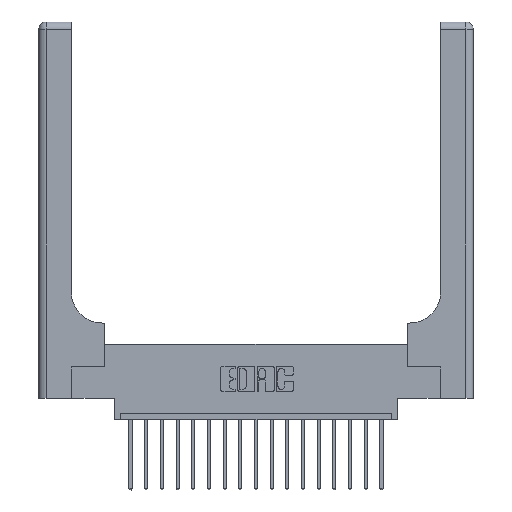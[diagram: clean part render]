
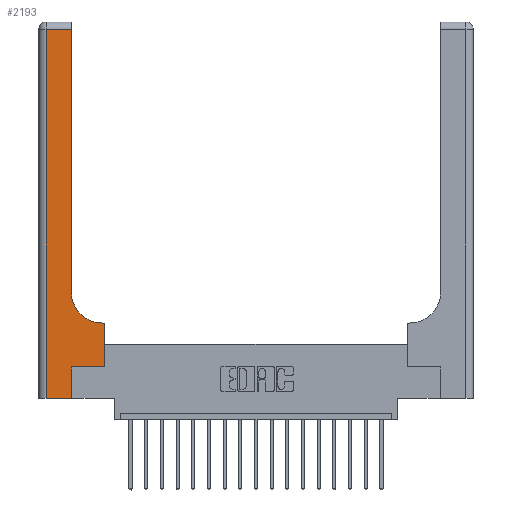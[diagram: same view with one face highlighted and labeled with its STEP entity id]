
A CAD part, top view. The second image highlights one B-rep face of the part: STEP entity #2193.
In plain terms, the highlighted planar face has unit normal (0, 0, 1).
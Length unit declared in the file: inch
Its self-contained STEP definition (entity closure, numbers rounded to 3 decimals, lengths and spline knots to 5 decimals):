
#45 = EDGE_CURVE ( 'NONE', #14187, #7645, #11312, .T. ) ;
#252 = CARTESIAN_POINT ( 'NONE',  ( 0.06, 3., 0.37 ) ) ;
#544 = EDGE_CURVE ( 'NONE', #1887, #4489, #12196, .T. ) ;
#926 = LINE ( 'NONE', #252, #4419 ) ;
#1723 = LINE ( 'NONE', #17283, #16121 ) ;
#1765 = EDGE_CURVE ( 'NONE', #5808, #10718, #11257, .T. ) ;
#1887 = VERTEX_POINT ( 'NONE', #8858 ) ;
#2193 = ADVANCED_FACE ( 'NONE', ( #14904 ), #18924, .F. ) ;
#2476 = CARTESIAN_POINT ( 'NONE',  ( 0.06, 2.94, 0.37 ) ) ;
#2919 = ORIENTED_EDGE ( 'NONE', *, *, #11813, .T. ) ;
#2943 = EDGE_CURVE ( 'NONE', #10911, #1887, #12102, .T. ) ;
#3172 = EDGE_CURVE ( 'NONE', #7645, #10911, #13008, .T. ) ;
#3522 = DIRECTION ( 'NONE',  ( 0., 1., 0. ) ) ;
#3630 = ORIENTED_EDGE ( 'NONE', *, *, #16964, .T. ) ;
#3651 = VECTOR ( 'NONE', #7905, 39.37008 ) ;
#3683 = CARTESIAN_POINT ( 'NONE',  ( 0.528, 0.25, 0.37 ) ) ;
#4224 = ORIENTED_EDGE ( 'NONE', *, *, #544, .T. ) ;
#4419 = VECTOR ( 'NONE', #13472, 39.37008 ) ;
#4489 = VERTEX_POINT ( 'NONE', #5322 ) ;
#4621 = VECTOR ( 'NONE', #13363, 39.37008 ) ;
#4865 = VECTOR ( 'NONE', #3522, 39.37008 ) ;
#4962 = CARTESIAN_POINT ( 'NONE',  ( 0.528, 0.25, 0.37 ) ) ;
#5295 = VERTEX_POINT ( 'NONE', #5803 ) ;
#5322 = CARTESIAN_POINT ( 'NONE',  ( 0.51, 0.6, 0.37 ) ) ;
#5636 = ORIENTED_EDGE ( 'NONE', *, *, #9263, .T. ) ;
#5675 = VECTOR ( 'NONE', #7975, 39.37008 ) ;
#5803 = CARTESIAN_POINT ( 'NONE',  ( 0.06, 0., 0.37 ) ) ;
#5808 = VERTEX_POINT ( 'NONE', #9165 ) ;
#6165 = ORIENTED_EDGE ( 'NONE', *, *, #45, .T. ) ;
#6620 = DIRECTION ( 'NONE',  ( -1., 0., 0. ) ) ;
#7645 = VERTEX_POINT ( 'NONE', #10426 ) ;
#7803 = ORIENTED_EDGE ( 'NONE', *, *, #2943, .T. ) ;
#7905 = DIRECTION ( 'NONE',  ( 1., 0., 0. ) ) ;
#7938 = EDGE_CURVE ( 'NONE', #5295, #14187, #12512, .T. ) ;
#7975 = DIRECTION ( 'NONE',  ( 0., 1., 0. ) ) ;
#7982 = CARTESIAN_POINT ( 'NONE',  ( 0.51, 0.85, 0.37 ) ) ;
#8212 = DIRECTION ( 'NONE',  ( -1., 0., 0. ) ) ;
#8539 = ORIENTED_EDGE ( 'NONE', *, *, #3172, .T. ) ;
#8858 = CARTESIAN_POINT ( 'NONE',  ( 0.528, 0.6, 0.37 ) ) ;
#9165 = CARTESIAN_POINT ( 'NONE',  ( 0.26, 2.94, 0.37 ) ) ;
#9263 = EDGE_CURVE ( 'NONE', #4489, #10471, #16848, .T. ) ;
#9624 = CARTESIAN_POINT ( 'NONE',  ( 0.265, 0., 0.37 ) ) ;
#10426 = CARTESIAN_POINT ( 'NONE',  ( 0.265, 0.25, 0.37 ) ) ;
#10471 = VERTEX_POINT ( 'NONE', #15401 ) ;
#10718 = VERTEX_POINT ( 'NONE', #2476 ) ;
#10729 = CARTESIAN_POINT ( 'NONE',  ( 0., 0., 0.37 ) ) ;
#10801 = DIRECTION ( 'NONE',  ( 0., 0., -1. ) ) ;
#10911 = VERTEX_POINT ( 'NONE', #3683 ) ;
#11257 = LINE ( 'NONE', #15588, #14703 ) ;
#11312 = LINE ( 'NONE', #18549, #5675 ) ;
#11475 = EDGE_LOOP ( 'NONE', ( #2919, #13630, #3630, #15937, #6165, #8539, #7803, #4224, #5636 ) ) ;
#11813 = EDGE_CURVE ( 'NONE', #10471, #5808, #1723, .T. ) ;
#12102 = LINE ( 'NONE', #4962, #4865 ) ;
#12196 = LINE ( 'NONE', #17188, #19127 ) ;
#12512 = LINE ( 'NONE', #10729, #3651 ) ;
#13008 = LINE ( 'NONE', #17756, #4621 ) ;
#13363 = DIRECTION ( 'NONE',  ( 1., 0., 0. ) ) ;
#13472 = DIRECTION ( 'NONE',  ( 0., -1., 0. ) ) ;
#13630 = ORIENTED_EDGE ( 'NONE', *, *, #1765, .T. ) ;
#13756 = DIRECTION ( 'NONE',  ( 1., 0., 0. ) ) ;
#14187 = VERTEX_POINT ( 'NONE', #9624 ) ;
#14703 = VECTOR ( 'NONE', #8212, 39.37008 ) ;
#14904 = FACE_OUTER_BOUND ( 'NONE', #11475, .T. ) ;
#15401 = CARTESIAN_POINT ( 'NONE',  ( 0.26, 0.85, 0.37 ) ) ;
#15588 = CARTESIAN_POINT ( 'NONE',  ( 0., 2.94, 0.37 ) ) ;
#15690 = AXIS2_PLACEMENT_3D ( 'NONE', #7982, #10801, #13756 ) ;
#15937 = ORIENTED_EDGE ( 'NONE', *, *, #7938, .T. ) ;
#16059 = DIRECTION ( 'NONE',  ( 0., 1., 0. ) ) ;
#16121 = VECTOR ( 'NONE', #16059, 39.37008 ) ;
#16276 = AXIS2_PLACEMENT_3D ( 'NONE', #17370, #17311, #18743 ) ;
#16848 = CIRCLE ( 'NONE', #15690, 0.25 ) ;
#16964 = EDGE_CURVE ( 'NONE', #10718, #5295, #926, .T. ) ;
#17188 = CARTESIAN_POINT ( 'NONE',  ( 0.26, 0.6, 0.37 ) ) ;
#17283 = CARTESIAN_POINT ( 'NONE',  ( 0.26, 3., 0.37 ) ) ;
#17311 = DIRECTION ( 'NONE',  ( 0., 0., -1. ) ) ;
#17370 = CARTESIAN_POINT ( 'NONE',  ( 0., 3., 0.37 ) ) ;
#17756 = CARTESIAN_POINT ( 'NONE',  ( 0.265, 0.25, 0.37 ) ) ;
#18549 = CARTESIAN_POINT ( 'NONE',  ( 0.265, 0., 0.37 ) ) ;
#18743 = DIRECTION ( 'NONE',  ( -1., 0., 0. ) ) ;
#18924 = PLANE ( 'NONE',  #16276 ) ;
#19127 = VECTOR ( 'NONE', #6620, 39.37008 ) ;
